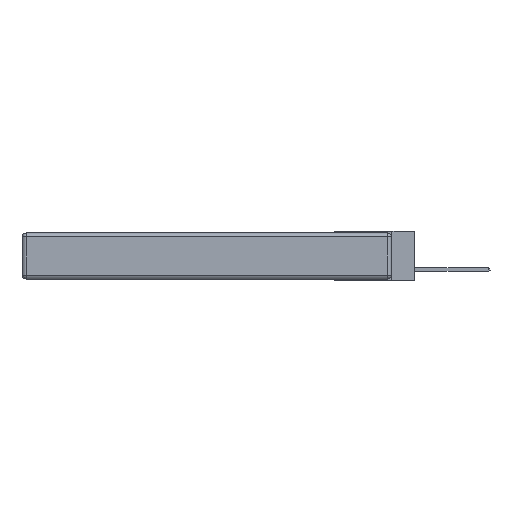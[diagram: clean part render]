
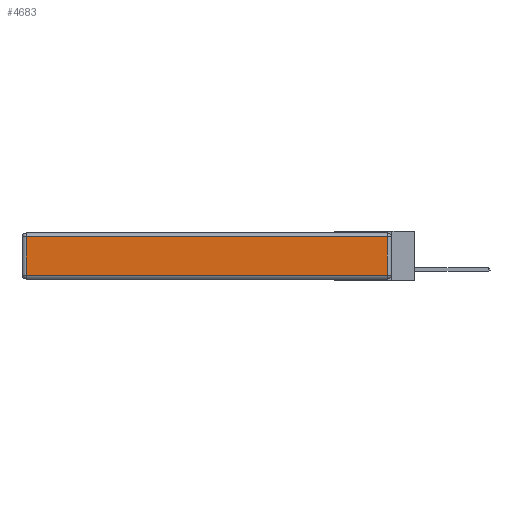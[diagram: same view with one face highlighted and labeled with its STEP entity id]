
A CAD part, left-side view. The second image highlights one B-rep face of the part: STEP entity #4683.
In plain terms, the highlighted planar face has unit normal (-1, 0, 0).
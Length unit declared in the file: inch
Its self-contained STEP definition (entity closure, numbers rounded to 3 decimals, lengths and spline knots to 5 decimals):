
#874 = DIRECTION ( 'NONE',  ( 0., 0., 1. ) ) ;
#1891 = EDGE_CURVE ( 'NONE', #25220, #14185, #16766, .T. ) ;
#2935 = DIRECTION ( 'NONE',  ( 0., 0., 1. ) ) ;
#4683 = ADVANCED_FACE ( 'NONE', ( #16295 ), #20215, .T. ) ;
#5252 = VERTEX_POINT ( 'NONE', #19966 ) ;
#6447 = VERTEX_POINT ( 'NONE', #17650 ) ;
#6860 = DIRECTION ( 'NONE',  ( 0., 0., -1. ) ) ;
#7468 = VECTOR ( 'NONE', #6860, 39.37008 ) ;
#8162 = EDGE_CURVE ( 'NONE', #5252, #25220, #20770, .T. ) ;
#8531 = CARTESIAN_POINT ( 'NONE',  ( 0., 0., -0.313 ) ) ;
#9942 = ORIENTED_EDGE ( 'NONE', *, *, #17240, .T. ) ;
#10916 = EDGE_LOOP ( 'NONE', ( #23276, #19525, #11568, #9942 ) ) ;
#11568 = ORIENTED_EDGE ( 'NONE', *, *, #30374, .T. ) ;
#14185 = VERTEX_POINT ( 'NONE', #29587 ) ;
#16295 = FACE_OUTER_BOUND ( 'NONE', #10916, .T. ) ;
#16766 = LINE ( 'NONE', #30824, #31203 ) ;
#16778 = DIRECTION ( 'NONE',  ( 0., 1., 0. ) ) ;
#17087 = CARTESIAN_POINT ( 'NONE',  ( 0., 2.72, -0.343 ) ) ;
#17240 = EDGE_CURVE ( 'NONE', #6447, #5252, #24587, .T. ) ;
#17650 = CARTESIAN_POINT ( 'NONE',  ( 0., 2.72, -0.03 ) ) ;
#19525 = ORIENTED_EDGE ( 'NONE', *, *, #1891, .T. ) ;
#19966 = CARTESIAN_POINT ( 'NONE',  ( 0., 2.72, -0.313 ) ) ;
#20215 = PLANE ( 'NONE',  #30046 ) ;
#20770 = LINE ( 'NONE', #8531, #26197 ) ;
#21042 = LINE ( 'NONE', #26470, #25718 ) ;
#22952 = CARTESIAN_POINT ( 'NONE',  ( 0., 0., -0.343 ) ) ;
#23276 = ORIENTED_EDGE ( 'NONE', *, *, #8162, .T. ) ;
#23365 = CARTESIAN_POINT ( 'NONE',  ( 0., 0.03, -0.313 ) ) ;
#24587 = LINE ( 'NONE', #17087, #7468 ) ;
#25036 = DIRECTION ( 'NONE',  ( -1., 0., 0. ) ) ;
#25220 = VERTEX_POINT ( 'NONE', #23365 ) ;
#25718 = VECTOR ( 'NONE', #16778, 39.37008 ) ;
#26197 = VECTOR ( 'NONE', #30394, 39.37008 ) ;
#26470 = CARTESIAN_POINT ( 'NONE',  ( 0., 2.75, -0.03 ) ) ;
#29587 = CARTESIAN_POINT ( 'NONE',  ( 0., 0.03, -0.03 ) ) ;
#30046 = AXIS2_PLACEMENT_3D ( 'NONE', #22952, #25036, #2935 ) ;
#30374 = EDGE_CURVE ( 'NONE', #14185, #6447, #21042, .T. ) ;
#30394 = DIRECTION ( 'NONE',  ( 0., -1., 0. ) ) ;
#30824 = CARTESIAN_POINT ( 'NONE',  ( 0., 0.03, -0.343 ) ) ;
#31203 = VECTOR ( 'NONE', #874, 39.37008 ) ;
